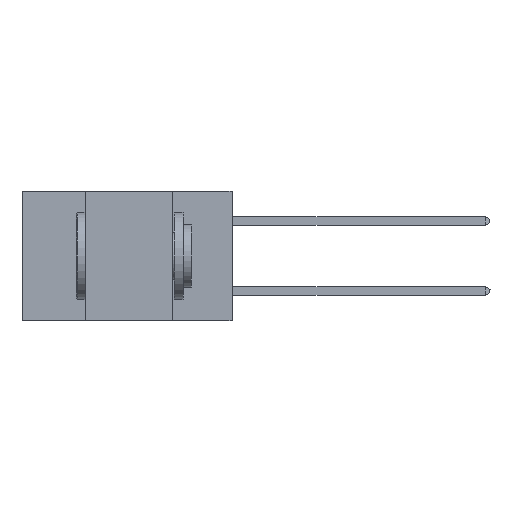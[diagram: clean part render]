
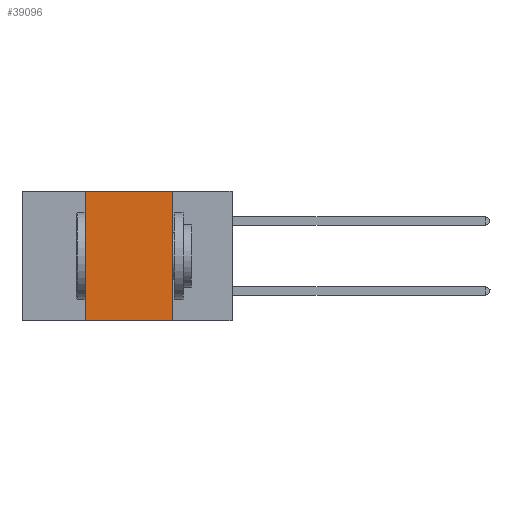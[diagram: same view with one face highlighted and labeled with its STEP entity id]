
A CAD part, left-side view. The second image highlights one B-rep face of the part: STEP entity #39096.
In plain terms, the highlighted planar face has unit normal (-1, 0, 0).
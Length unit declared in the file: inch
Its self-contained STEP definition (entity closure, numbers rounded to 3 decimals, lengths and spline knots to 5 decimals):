
#634 = VECTOR ( 'NONE', #15184, 39.37008 ) ;
#1769 = DIRECTION ( 'NONE',  ( 1., 0., 0. ) ) ;
#2820 = CARTESIAN_POINT ( 'NONE',  ( 0., 0.6, -0.37 ) ) ;
#2843 = ORIENTED_EDGE ( 'NONE', *, *, #19924, .F. ) ;
#3504 = FACE_OUTER_BOUND ( 'NONE', #8551, .T. ) ;
#3802 = EDGE_CURVE ( 'NONE', #34727, #13868, #34811, .T. ) ;
#7133 = ORIENTED_EDGE ( 'NONE', *, *, #36787, .F. ) ;
#8551 = EDGE_LOOP ( 'NONE', ( #22678, #2843, #7133, #35954 ) ) ;
#9060 = VECTOR ( 'NONE', #24924, 39.37008 ) ;
#11745 = EDGE_CURVE ( 'NONE', #20257, #13868, #41739, .T. ) ;
#13868 = VERTEX_POINT ( 'NONE', #34111 ) ;
#15184 = DIRECTION ( 'NONE',  ( 0., -1., 0. ) ) ;
#15391 = AXIS2_PLACEMENT_3D ( 'NONE', #28037, #1769, #21284 ) ;
#16131 = VERTEX_POINT ( 'NONE', #19685 ) ;
#16629 = CARTESIAN_POINT ( 'NONE',  ( 0., 0.17, 0. ) ) ;
#17583 = CARTESIAN_POINT ( 'NONE',  ( 0., 0.42, 0. ) ) ;
#19685 = CARTESIAN_POINT ( 'NONE',  ( 0., 0.42, 0. ) ) ;
#19924 = EDGE_CURVE ( 'NONE', #16131, #20257, #24056, .T. ) ;
#20257 = VERTEX_POINT ( 'NONE', #16629 ) ;
#21284 = DIRECTION ( 'NONE',  ( 0., 0., -1. ) ) ;
#22678 = ORIENTED_EDGE ( 'NONE', *, *, #11745, .F. ) ;
#24056 = LINE ( 'NONE', #35129, #9060 ) ;
#24924 = DIRECTION ( 'NONE',  ( 0., -1., 0. ) ) ;
#25246 = CARTESIAN_POINT ( 'NONE',  ( 0., 0.17, 0. ) ) ;
#25586 = VECTOR ( 'NONE', #31934, 39.37008 ) ;
#27889 = PLANE ( 'NONE',  #15391 ) ;
#28037 = CARTESIAN_POINT ( 'NONE',  ( 0., 0.6, 0. ) ) ;
#31934 = DIRECTION ( 'NONE',  ( 0., 0., -1. ) ) ;
#33224 = VECTOR ( 'NONE', #36877, 39.37008 ) ;
#34111 = CARTESIAN_POINT ( 'NONE',  ( 0., 0.17, -0.37 ) ) ;
#34727 = VERTEX_POINT ( 'NONE', #37643 ) ;
#34811 = LINE ( 'NONE', #2820, #634 ) ;
#35129 = CARTESIAN_POINT ( 'NONE',  ( 0., 0.6, 0. ) ) ;
#35954 = ORIENTED_EDGE ( 'NONE', *, *, #3802, .T. ) ;
#36787 = EDGE_CURVE ( 'NONE', #34727, #16131, #42056, .T. ) ;
#36877 = DIRECTION ( 'NONE',  ( 0., 0., 1. ) ) ;
#37643 = CARTESIAN_POINT ( 'NONE',  ( 0., 0.42, -0.37 ) ) ;
#39096 = ADVANCED_FACE ( 'NONE', ( #3504 ), #27889, .F. ) ;
#41739 = LINE ( 'NONE', #25246, #25586 ) ;
#42056 = LINE ( 'NONE', #17583, #33224 ) ;
